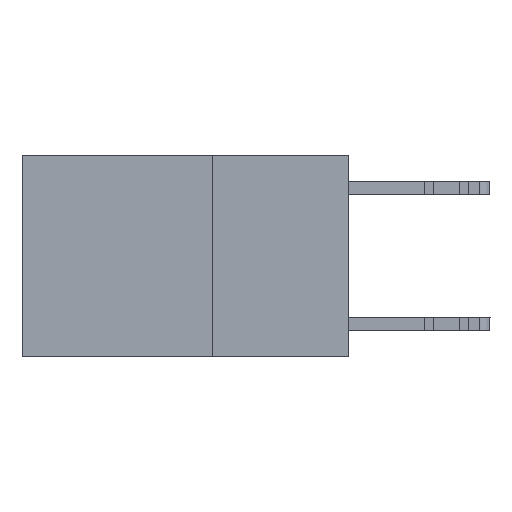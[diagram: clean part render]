
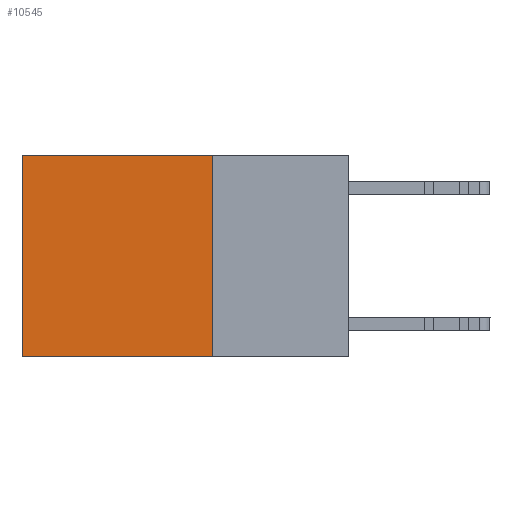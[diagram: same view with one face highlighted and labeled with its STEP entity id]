
A CAD part, left-side view. The second image highlights one B-rep face of the part: STEP entity #10545.
In plain terms, the highlighted planar face has unit normal (-1, 0, 0).
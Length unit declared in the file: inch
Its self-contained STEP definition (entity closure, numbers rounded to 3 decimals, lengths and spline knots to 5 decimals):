
#1053 = CARTESIAN_POINT ( 'NONE',  ( 0.2625, 0.25, 0. ) ) ;
#1453 = VERTEX_POINT ( 'NONE', #7729 ) ;
#4506 = AXIS2_PLACEMENT_3D ( 'NONE', #6378, #6190, #6117 ) ;
#4955 = EDGE_CURVE ( 'NONE', #11872, #1453, #19345, .T. ) ;
#6117 = DIRECTION ( 'NONE',  ( 0., 0., -1. ) ) ;
#6190 = DIRECTION ( 'NONE',  ( 1., 0., 0. ) ) ;
#6378 = CARTESIAN_POINT ( 'NONE',  ( 0.2625, 0.25, 0. ) ) ;
#6618 = DIRECTION ( 'NONE',  ( 0., 1., 0. ) ) ;
#7729 = CARTESIAN_POINT ( 'NONE',  ( 0.2625, 0.6, -0.37 ) ) ;
#8022 = EDGE_LOOP ( 'NONE', ( #27377, #9382, #16753, #12847 ) ) ;
#8358 = VECTOR ( 'NONE', #28991, 39.37008 ) ;
#9191 = LINE ( 'NONE', #1053, #8358 ) ;
#9382 = ORIENTED_EDGE ( 'NONE', *, *, #27030, .F. ) ;
#10545 = ADVANCED_FACE ( 'NONE', ( #10988 ), #11816, .F. ) ;
#10594 = EDGE_CURVE ( 'NONE', #18565, #11706, #9191, .T. ) ;
#10901 = DIRECTION ( 'NONE',  ( 0., 1., 0. ) ) ;
#10988 = FACE_OUTER_BOUND ( 'NONE', #8022, .T. ) ;
#11057 = CARTESIAN_POINT ( 'NONE',  ( 0.2625, 0.25, 0. ) ) ;
#11349 = CARTESIAN_POINT ( 'NONE',  ( 0.2625, 0.25, -0.37 ) ) ;
#11706 = VERTEX_POINT ( 'NONE', #25109 ) ;
#11816 = PLANE ( 'NONE',  #4506 ) ;
#11872 = VERTEX_POINT ( 'NONE', #20338 ) ;
#12275 = EDGE_CURVE ( 'NONE', #18565, #11872, #16184, .T. ) ;
#12451 = LINE ( 'NONE', #11349, #17334 ) ;
#12847 = ORIENTED_EDGE ( 'NONE', *, *, #12275, .T. ) ;
#15446 = VECTOR ( 'NONE', #10901, 39.37008 ) ;
#16184 = LINE ( 'NONE', #11057, #15446 ) ;
#16753 = ORIENTED_EDGE ( 'NONE', *, *, #10594, .F. ) ;
#17334 = VECTOR ( 'NONE', #6618, 39.37008 ) ;
#18565 = VERTEX_POINT ( 'NONE', #30733 ) ;
#19318 = VECTOR ( 'NONE', #30493, 39.37008 ) ;
#19345 = LINE ( 'NONE', #23323, #19318 ) ;
#20338 = CARTESIAN_POINT ( 'NONE',  ( 0.2625, 0.6, 0. ) ) ;
#23323 = CARTESIAN_POINT ( 'NONE',  ( 0.2625, 0.6, 0. ) ) ;
#25109 = CARTESIAN_POINT ( 'NONE',  ( 0.2625, 0.25, -0.37 ) ) ;
#27030 = EDGE_CURVE ( 'NONE', #11706, #1453, #12451, .T. ) ;
#27377 = ORIENTED_EDGE ( 'NONE', *, *, #4955, .T. ) ;
#28991 = DIRECTION ( 'NONE',  ( 0., 0., -1. ) ) ;
#30493 = DIRECTION ( 'NONE',  ( 0., 0., -1. ) ) ;
#30733 = CARTESIAN_POINT ( 'NONE',  ( 0.2625, 0.25, 0. ) ) ;
